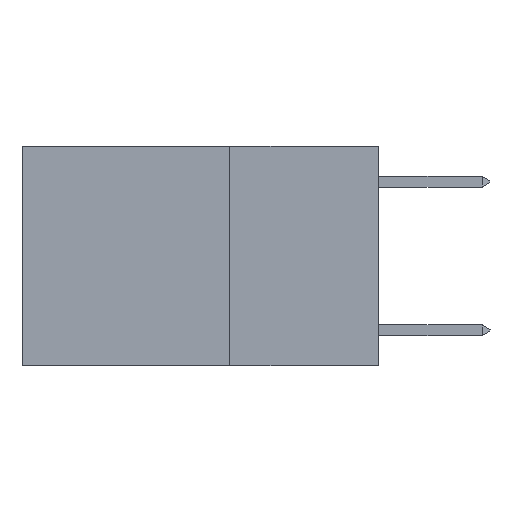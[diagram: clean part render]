
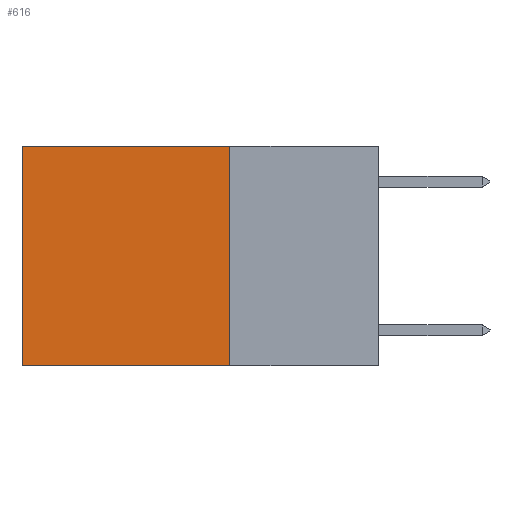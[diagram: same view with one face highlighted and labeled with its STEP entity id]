
A CAD part, left-side view. The second image highlights one B-rep face of the part: STEP entity #616.
In plain terms, the highlighted planar face has unit normal (-1, 0, 0).
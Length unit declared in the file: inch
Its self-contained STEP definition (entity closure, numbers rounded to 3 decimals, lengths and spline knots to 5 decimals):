
#3 = DIRECTION ( 'NONE',  ( 0., 0., -1. ) ) ;
#531 = CARTESIAN_POINT ( 'NONE',  ( 0.2625, 0.6, -0.37 ) ) ;
#577 = FACE_OUTER_BOUND ( 'NONE', #9704, .T. ) ;
#616 = ADVANCED_FACE ( 'NONE', ( #577 ), #9713, .F. ) ;
#1223 = EDGE_CURVE ( 'NONE', #24778, #14340, #8973, .T. ) ;
#2822 = CARTESIAN_POINT ( 'NONE',  ( 0.2625, 0.25, -0.37 ) ) ;
#3156 = VECTOR ( 'NONE', #21027, 39.37008 ) ;
#4835 = CARTESIAN_POINT ( 'NONE',  ( 0.2625, 0.25, 0. ) ) ;
#4870 = ORIENTED_EDGE ( 'NONE', *, *, #24218, .F. ) ;
#7004 = VERTEX_POINT ( 'NONE', #2822 ) ;
#7023 = EDGE_CURVE ( 'NONE', #24778, #7004, #20229, .T. ) ;
#7478 = ORIENTED_EDGE ( 'NONE', *, *, #11985, .T. ) ;
#8350 = ORIENTED_EDGE ( 'NONE', *, *, #1223, .T. ) ;
#8480 = ORIENTED_EDGE ( 'NONE', *, *, #7023, .F. ) ;
#8973 = LINE ( 'NONE', #19117, #3156 ) ;
#9051 = CARTESIAN_POINT ( 'NONE',  ( 0.2625, 0.6, 0. ) ) ;
#9704 = EDGE_LOOP ( 'NONE', ( #7478, #4870, #8480, #8350 ) ) ;
#9713 = PLANE ( 'NONE',  #14608 ) ;
#11739 = DIRECTION ( 'NONE',  ( 1., 0., 0. ) ) ;
#11985 = EDGE_CURVE ( 'NONE', #14340, #14931, #12780, .T. ) ;
#12599 = DIRECTION ( 'NONE',  ( 0., 0., -1. ) ) ;
#12780 = LINE ( 'NONE', #9051, #21850 ) ;
#13436 = CARTESIAN_POINT ( 'NONE',  ( 0.2625, 0.25, -0.37 ) ) ;
#14340 = VERTEX_POINT ( 'NONE', #23278 ) ;
#14608 = AXIS2_PLACEMENT_3D ( 'NONE', #21381, #11739, #3 ) ;
#14931 = VERTEX_POINT ( 'NONE', #531 ) ;
#15086 = VECTOR ( 'NONE', #12599, 39.37008 ) ;
#18985 = VECTOR ( 'NONE', #24941, 39.37008 ) ;
#19117 = CARTESIAN_POINT ( 'NONE',  ( 0.2625, 0.25, 0. ) ) ;
#19369 = CARTESIAN_POINT ( 'NONE',  ( 0.2625, 0.25, 0. ) ) ;
#20229 = LINE ( 'NONE', #4835, #15086 ) ;
#21027 = DIRECTION ( 'NONE',  ( 0., 1., 0. ) ) ;
#21381 = CARTESIAN_POINT ( 'NONE',  ( 0.2625, 0.25, 0. ) ) ;
#21850 = VECTOR ( 'NONE', #24445, 39.37008 ) ;
#23278 = CARTESIAN_POINT ( 'NONE',  ( 0.2625, 0.6, 0. ) ) ;
#24039 = LINE ( 'NONE', #13436, #18985 ) ;
#24218 = EDGE_CURVE ( 'NONE', #7004, #14931, #24039, .T. ) ;
#24445 = DIRECTION ( 'NONE',  ( 0., 0., -1. ) ) ;
#24778 = VERTEX_POINT ( 'NONE', #19369 ) ;
#24941 = DIRECTION ( 'NONE',  ( 0., 1., 0. ) ) ;
